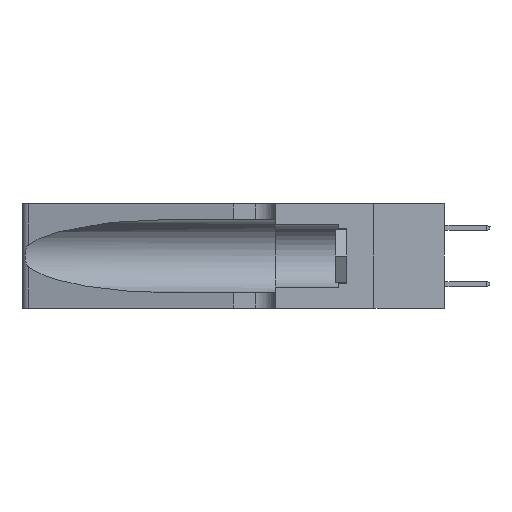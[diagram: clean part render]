
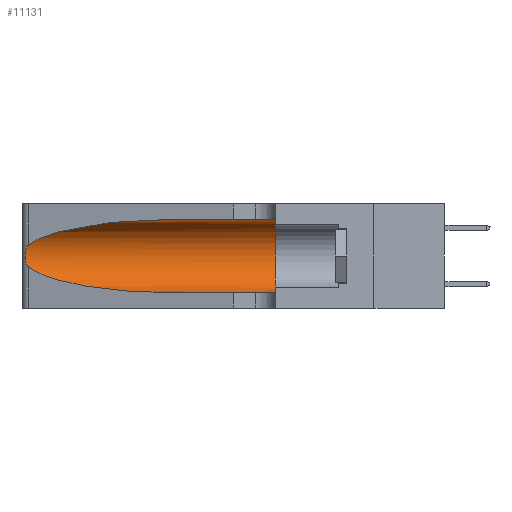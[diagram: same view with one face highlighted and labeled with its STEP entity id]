
A CAD part, left-side view. The second image highlights one B-rep face of the part: STEP entity #11131.
In plain terms, the highlighted cylindrical face has radius 3.308 mm (diameter 6.617 mm), a partial arc.
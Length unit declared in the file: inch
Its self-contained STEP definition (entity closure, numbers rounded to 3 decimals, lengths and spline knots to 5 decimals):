
#726 = ORIENTED_EDGE ( 'NONE', *, *, #34059, .F. ) ;
#830 = DIRECTION ( 'NONE',  ( 0., -1., 0. ) ) ;
#1435 = CARTESIAN_POINT ( 'NONE',  ( 0.25487, 1.22718, 0.14631 ) ) ;
#2552 = CARTESIAN_POINT ( 'NONE',  ( 0.1305, 0.35, 0.31525 ) ) ;
#3222 = B_SPLINE_CURVE_WITH_KNOTS ( 'NONE', 3,
 ( #12643, #12906, #4481, #27534, #4353, #13172, #27407, #9945, #24829, #30446, #36052, #33263, #7269, #21639 ),
 .UNSPECIFIED., .F., .F.,
 ( 4, 2, 2, 2, 2, 2, 4 ),
 ( 0., 0.00027, 0.00053, 0.00107, 0.0016, 0.00187, 0.00214 ),
 .UNSPECIFIED. ) ;
#4353 = CARTESIAN_POINT ( 'NONE',  ( 0.25854, 1.2359, 0.20912 ) ) ;
#4481 = CARTESIAN_POINT ( 'NONE',  ( 0.25639, 1.23184, 0.21858 ) ) ;
#4599 = CARTESIAN_POINT ( 'NONE',  ( 0.1305, 0.72297, 0.31525 ) ) ;
#6135 = LINE ( 'NONE', #24100, #22148 ) ;
#6348 = CIRCLE ( 'NONE', #19163, 0.13025 ) ;
#6893 = LINE ( 'NONE', #32108, #13342 ) ;
#7095 = CARTESIAN_POINT ( 'NONE',  ( 0.1305, 0.72297, 0.05475 ) ) ;
#7269 = CARTESIAN_POINT ( 'NONE',  ( 0.25555, 1.22993, 0.14849 ) ) ;
#8301 = DIRECTION ( 'NONE',  ( 0., -1., 0. ) ) ;
#8659 = EDGE_CURVE ( 'NONE', #22464, #27823, #6135, .T. ) ;
#9333 = EDGE_LOOP ( 'NONE', ( #32612, #13343, #11353, #30776, #16551, #726 ) ) ;
#9945 = CARTESIAN_POINT ( 'NONE',  ( 0.26075, 1.23896, 0.178 ) ) ;
#10200 = EDGE_CURVE ( 'NONE', #22227, #23626, #16296, .T. ) ;
#11131 = ADVANCED_FACE ( 'NONE', ( #30656 ), #23327, .F. ) ;
#11353 = ORIENTED_EDGE ( 'NONE', *, *, #22718, .T. ) ;
#12643 = CARTESIAN_POINT ( 'NONE',  ( 0.25487, 1.22718, 0.22369 ) ) ;
#12906 = CARTESIAN_POINT ( 'NONE',  ( 0.25555, 1.22994, 0.2215 ) ) ;
#13172 = CARTESIAN_POINT ( 'NONE',  ( 0.26018, 1.23835, 0.19895 ) ) ;
#13342 = VECTOR ( 'NONE', #8301, 39.37008 ) ;
#13343 = ORIENTED_EDGE ( 'NONE', *, *, #27433, .T. ) ;
#13681 = CARTESIAN_POINT ( 'NONE',  ( 0.25487, 1.22718, 0.22369 ) ) ;
#13962 = CARTESIAN_POINT ( 'NONE',  ( 0.25487, 1.22718, 0.22369 ) ) ;
#16296 =( BOUNDED_CURVE ( )  B_SPLINE_CURVE ( 3, ( #37082, #19577, #30940, #13681 ),
 .UNSPECIFIED., .F., .F. ) 
 B_SPLINE_CURVE_WITH_KNOTS ( ( 4, 4 ),
 ( 1.5708, 2.84003 ),
 .UNSPECIFIED. ) 
 CURVE ( )  GEOMETRIC_REPRESENTATION_ITEM ( )  RATIONAL_B_SPLINE_CURVE ( ( 1., 0.87, 0.87, 1. ) ) 
 REPRESENTATION_ITEM ( '' )  );
#16323 = CARTESIAN_POINT ( 'NONE',  ( 0.1305, 0.35, 0.185 ) ) ;
#16551 = ORIENTED_EDGE ( 'NONE', *, *, #19539, .F. ) ;
#16668 = DIRECTION ( 'NONE',  ( 0., -1., 0. ) ) ;
#17979 = CARTESIAN_POINT ( 'NONE',  ( 0.1305, 0.72297, 0.05475 ) ) ;
#19163 = AXIS2_PLACEMENT_3D ( 'NONE', #16323, #21739, #34004 ) ;
#19539 = EDGE_CURVE ( 'NONE', #33850, #27823, #6348, .T. ) ;
#19577 = CARTESIAN_POINT ( 'NONE',  ( 0.18966, 0.96281, 0.31525 ) ) ;
#21639 = CARTESIAN_POINT ( 'NONE',  ( 0.25487, 1.22718, 0.14631 ) ) ;
#21709 = CARTESIAN_POINT ( 'NONE',  ( 0.25487, 1.22718, 0.14631 ) ) ;
#21739 = DIRECTION ( 'NONE',  ( 0., 1., 0. ) ) ;
#22148 = VECTOR ( 'NONE', #830, 39.37008 ) ;
#22227 = VERTEX_POINT ( 'NONE', #4599 ) ;
#22464 = VERTEX_POINT ( 'NONE', #17979 ) ;
#22718 = EDGE_CURVE ( 'NONE', #32352, #22464, #33435, .T. ) ;
#23327 = CYLINDRICAL_SURFACE ( 'NONE', #34209, 0.13025 ) ;
#23626 = VERTEX_POINT ( 'NONE', #13962 ) ;
#24100 = CARTESIAN_POINT ( 'NONE',  ( 0.1305, 1.61858, 0.05475 ) ) ;
#24829 = CARTESIAN_POINT ( 'NONE',  ( 0.26017, 1.23833, 0.17102 ) ) ;
#26114 = CARTESIAN_POINT ( 'NONE',  ( 0.1305, 0.35, 0.05475 ) ) ;
#27407 = CARTESIAN_POINT ( 'NONE',  ( 0.26075, 1.23896, 0.19203 ) ) ;
#27433 = EDGE_CURVE ( 'NONE', #23626, #32352, #3222, .T. ) ;
#27534 = CARTESIAN_POINT ( 'NONE',  ( 0.25787, 1.23484, 0.2124 ) ) ;
#27823 = VERTEX_POINT ( 'NONE', #26114 ) ;
#30446 = CARTESIAN_POINT ( 'NONE',  ( 0.25856, 1.23593, 0.16098 ) ) ;
#30519 = CARTESIAN_POINT ( 'NONE',  ( 0.18966, 0.96281, 0.05475 ) ) ;
#30656 = FACE_OUTER_BOUND ( 'NONE', #9333, .T. ) ;
#30776 = ORIENTED_EDGE ( 'NONE', *, *, #8659, .T. ) ;
#30940 = CARTESIAN_POINT ( 'NONE',  ( 0.2373, 1.15595, 0.28018 ) ) ;
#32108 = CARTESIAN_POINT ( 'NONE',  ( 0.1305, 1.61858, 0.31525 ) ) ;
#32352 = VERTEX_POINT ( 'NONE', #1435 ) ;
#32612 = ORIENTED_EDGE ( 'NONE', *, *, #10200, .T. ) ;
#33263 = CARTESIAN_POINT ( 'NONE',  ( 0.25639, 1.23186, 0.15144 ) ) ;
#33435 =( BOUNDED_CURVE ( )  B_SPLINE_CURVE ( 3, ( #21709, #36259, #30519, #7095 ),
 .UNSPECIFIED., .F., .F. ) 
 B_SPLINE_CURVE_WITH_KNOTS ( ( 4, 4 ),
 ( 3.44316, 4.71239 ),
 .UNSPECIFIED. ) 
 CURVE ( )  GEOMETRIC_REPRESENTATION_ITEM ( )  RATIONAL_B_SPLINE_CURVE ( ( 1., 0.87, 0.87, 1. ) ) 
 REPRESENTATION_ITEM ( '' )  );
#33850 = VERTEX_POINT ( 'NONE', #2552 ) ;
#34004 = DIRECTION ( 'NONE',  ( 0., 0., 1. ) ) ;
#34059 = EDGE_CURVE ( 'NONE', #22227, #33850, #6893, .T. ) ;
#34209 = AXIS2_PLACEMENT_3D ( 'NONE', #37538, #16668, #37138 ) ;
#36052 = CARTESIAN_POINT ( 'NONE',  ( 0.25789, 1.23486, 0.15765 ) ) ;
#36259 = CARTESIAN_POINT ( 'NONE',  ( 0.2373, 1.15595, 0.08982 ) ) ;
#37082 = CARTESIAN_POINT ( 'NONE',  ( 0.1305, 0.72297, 0.31525 ) ) ;
#37138 = DIRECTION ( 'NONE',  ( 0., 0., -1. ) ) ;
#37538 = CARTESIAN_POINT ( 'NONE',  ( 0.1305, 1.61858, 0.185 ) ) ;
